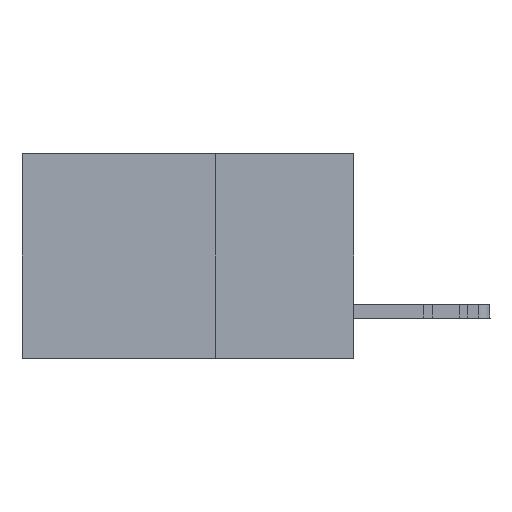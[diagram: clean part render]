
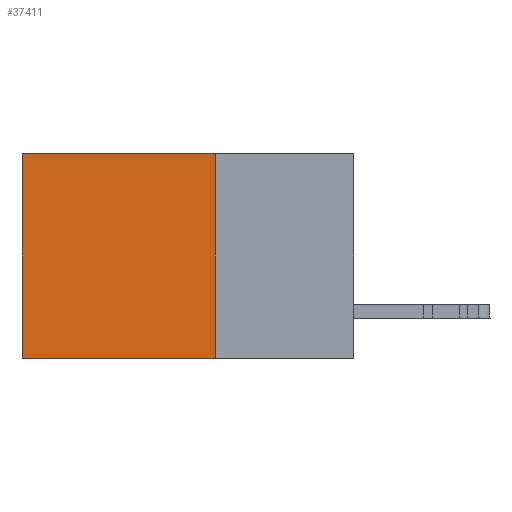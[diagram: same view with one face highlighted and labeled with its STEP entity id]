
A CAD part, left-side view. The second image highlights one B-rep face of the part: STEP entity #37411.
In plain terms, the highlighted planar face has unit normal (-1, 0, 0).
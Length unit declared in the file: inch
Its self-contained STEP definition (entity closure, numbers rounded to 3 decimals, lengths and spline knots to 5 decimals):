
#436 = DIRECTION ( 'NONE',  ( 0., 0., -1. ) ) ;
#695 = CARTESIAN_POINT ( 'NONE',  ( 0.2875, 0.25, 0. ) ) ;
#1137 = EDGE_CURVE ( 'NONE', #37006, #22663, #23382, .T. ) ;
#1746 = CARTESIAN_POINT ( 'NONE',  ( 0.2875, 0.6, 0. ) ) ;
#3254 = EDGE_CURVE ( 'NONE', #27954, #37006, #28190, .T. ) ;
#4939 = CARTESIAN_POINT ( 'NONE',  ( 0.2875, 0.25, 0. ) ) ;
#5088 = LINE ( 'NONE', #4939, #29123 ) ;
#5727 = DIRECTION ( 'NONE',  ( 0., 0., -1. ) ) ;
#6931 = PLANE ( 'NONE',  #25335 ) ;
#6953 = FACE_OUTER_BOUND ( 'NONE', #27970, .T. ) ;
#8925 = CARTESIAN_POINT ( 'NONE',  ( 0.2875, 0.25, -0.37 ) ) ;
#9207 = LINE ( 'NONE', #8925, #33291 ) ;
#12774 = ORIENTED_EDGE ( 'NONE', *, *, #34512, .F. ) ;
#13050 = VECTOR ( 'NONE', #5727, 39.37008 ) ;
#14656 = DIRECTION ( 'NONE',  ( 0., 0., -1. ) ) ;
#14767 = EDGE_CURVE ( 'NONE', #27954, #16739, #5088, .T. ) ;
#14806 = CARTESIAN_POINT ( 'NONE',  ( 0.2875, 0.6, 0. ) ) ;
#15909 = DIRECTION ( 'NONE',  ( 0., 1., 0. ) ) ;
#16739 = VERTEX_POINT ( 'NONE', #35304 ) ;
#17965 = DIRECTION ( 'NONE',  ( 0., 1., 0. ) ) ;
#19675 = DIRECTION ( 'NONE',  ( 1., 0., 0. ) ) ;
#20817 = CARTESIAN_POINT ( 'NONE',  ( 0.2875, 0.25, 0. ) ) ;
#22663 = VERTEX_POINT ( 'NONE', #23613 ) ;
#23382 = LINE ( 'NONE', #14806, #13050 ) ;
#23613 = CARTESIAN_POINT ( 'NONE',  ( 0.2875, 0.6, -0.37 ) ) ;
#25335 = AXIS2_PLACEMENT_3D ( 'NONE', #695, #19675, #436 ) ;
#27954 = VERTEX_POINT ( 'NONE', #29994 ) ;
#27970 = EDGE_LOOP ( 'NONE', ( #29242, #12774, #30559, #28558 ) ) ;
#28190 = LINE ( 'NONE', #20817, #29573 ) ;
#28558 = ORIENTED_EDGE ( 'NONE', *, *, #3254, .T. ) ;
#29123 = VECTOR ( 'NONE', #14656, 39.37008 ) ;
#29242 = ORIENTED_EDGE ( 'NONE', *, *, #1137, .T. ) ;
#29573 = VECTOR ( 'NONE', #17965, 39.37008 ) ;
#29994 = CARTESIAN_POINT ( 'NONE',  ( 0.2875, 0.25, 0. ) ) ;
#30559 = ORIENTED_EDGE ( 'NONE', *, *, #14767, .F. ) ;
#33291 = VECTOR ( 'NONE', #15909, 39.37008 ) ;
#34512 = EDGE_CURVE ( 'NONE', #16739, #22663, #9207, .T. ) ;
#35304 = CARTESIAN_POINT ( 'NONE',  ( 0.2875, 0.25, -0.37 ) ) ;
#37006 = VERTEX_POINT ( 'NONE', #1746 ) ;
#37411 = ADVANCED_FACE ( 'NONE', ( #6953 ), #6931, .F. ) ;
